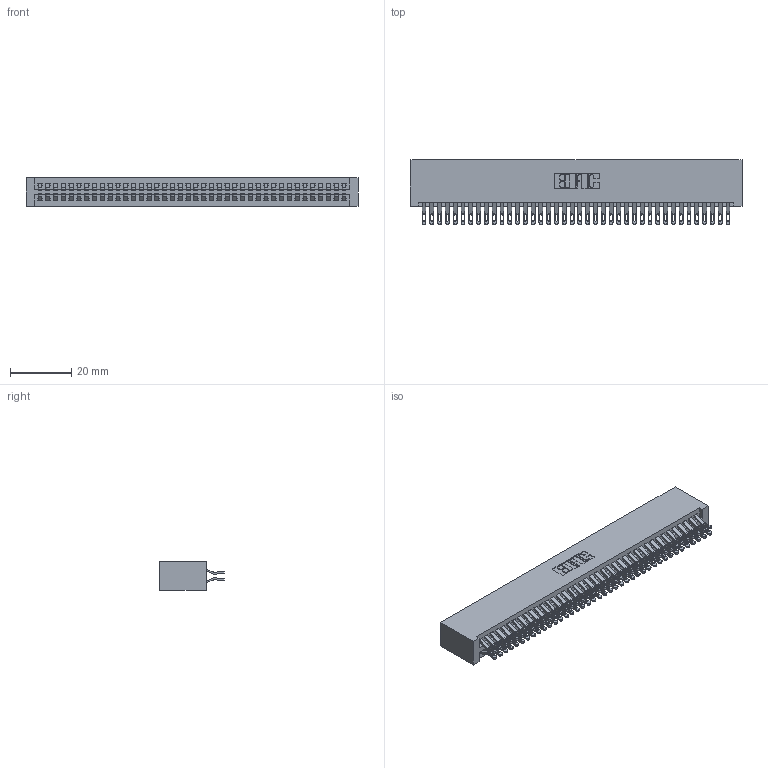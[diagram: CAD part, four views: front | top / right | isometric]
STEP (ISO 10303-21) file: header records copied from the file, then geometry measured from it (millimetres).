
FILE_DESCRIPTION (( 'STEP AP203' ), '1' );
FILE_NAME ('345-080-555-201.STEP', '2019-10-31T19:59:51', ( '' ), ( '' ), 'SwSTEP 2.0', 'SolidWorks 2016', '' );
FILE_SCHEMA (( 'CONFIG_CONTROL_DESIGN' ));
Length unit declared in the file: inch
Products named in the file (3): 345-080-555-201; 345-292-001_555 Tail; 345 Part_No Mounting Lugs
Assembly tree (81 placements, depth 2):
  345-080-555-201
    345 Part_No Mounting Lugs
    345-292-001_555 Tail  x80
Bounding box: 108.2 x 21.13 x 9.4 mm (x, y, z)
Volume: 11340.4 mm3; surface area: 17834.7 mm2
Topology: 81 solids, 81 shells, 4598 faces, 14477 edges, 9650 vertices
Faces by surface type: plane 2556, cylinder 2042
Entity records: 31703 total; most frequent: CARTESIAN_POINT 5350, ORIENTED_EDGE 5254, DIRECTION 4683, EDGE_CURVE 2627, VECTOR 2323, LINE 2323, VERTEX_POINT 1750, AXIS2_PLACEMENT_3D 1180
